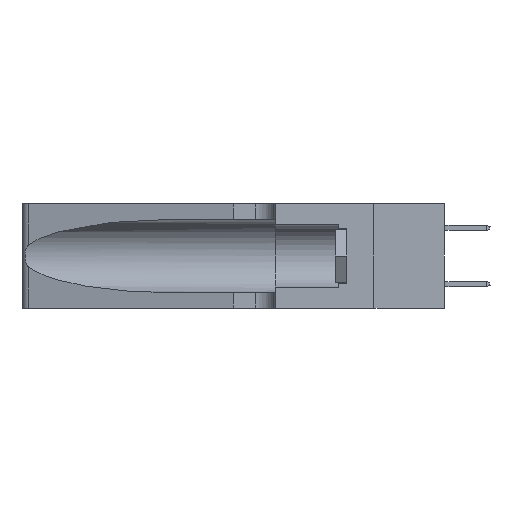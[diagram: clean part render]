
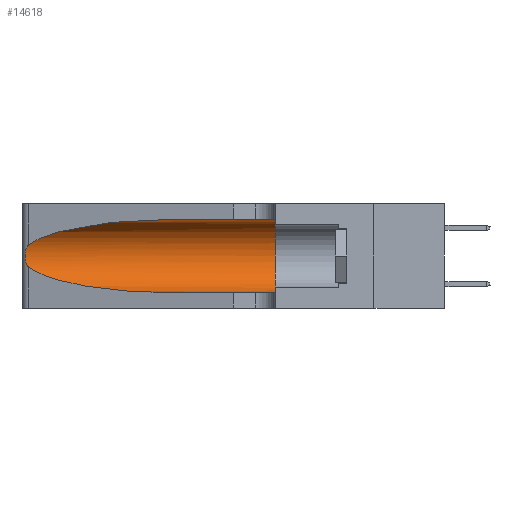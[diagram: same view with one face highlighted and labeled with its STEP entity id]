
A CAD part, left-side view. The second image highlights one B-rep face of the part: STEP entity #14618.
In plain terms, the highlighted cylindrical face has radius 3.308 mm (diameter 6.617 mm), a partial arc.
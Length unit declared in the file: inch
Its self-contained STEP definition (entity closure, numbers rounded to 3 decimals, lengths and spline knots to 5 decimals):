
#672 = CYLINDRICAL_SURFACE ( 'NONE', #8063, 0.13025 ) ;
#732 = CARTESIAN_POINT ( 'NONE',  ( 0.25789, 1.23486, 0.15765 ) ) ;
#1473 = VERTEX_POINT ( 'NONE', #19473 ) ;
#2436 = CARTESIAN_POINT ( 'NONE',  ( 0.25487, 1.22718, 0.22369 ) ) ;
#3015 = ORIENTED_EDGE ( 'NONE', *, *, #11778, .T. ) ;
#3495 = CARTESIAN_POINT ( 'NONE',  ( 0.25555, 1.22993, 0.14849 ) ) ;
#3875 = LINE ( 'NONE', #29066, #17285 ) ;
#5190 = ORIENTED_EDGE ( 'NONE', *, *, #21490, .F. ) ;
#5998 = ORIENTED_EDGE ( 'NONE', *, *, #27264, .F. ) ;
#6663 = VERTEX_POINT ( 'NONE', #19026 ) ;
#7786 = CARTESIAN_POINT ( 'NONE',  ( 0.1305, 0.72297, 0.05475 ) ) ;
#7862 = EDGE_CURVE ( 'NONE', #17977, #1473, #10092, .T. ) ;
#8063 = AXIS2_PLACEMENT_3D ( 'NONE', #27535, #8978, #30194 ) ;
#8717 = CIRCLE ( 'NONE', #23995, 0.13025 ) ;
#8726 = CARTESIAN_POINT ( 'NONE',  ( 0.25555, 1.22994, 0.2215 ) ) ;
#8837 = CARTESIAN_POINT ( 'NONE',  ( 0.25787, 1.23484, 0.2124 ) ) ;
#8978 = DIRECTION ( 'NONE',  ( 0., -1., 0. ) ) ;
#10092 =( BOUNDED_CURVE ( )  B_SPLINE_CURVE ( 3, ( #31660, #34314, #18511, #2436 ),
 .UNSPECIFIED., .F., .T. ) 
 B_SPLINE_CURVE_WITH_KNOTS ( ( 4, 4 ),
 ( 1.5708, 2.84003 ),
 .UNSPECIFIED. ) 
 CURVE ( )  GEOMETRIC_REPRESENTATION_ITEM ( )  RATIONAL_B_SPLINE_CURVE ( ( 1., 0.87, 0.87, 1. ) ) 
 REPRESENTATION_ITEM ( '' )  );
#10365 = ORIENTED_EDGE ( 'NONE', *, *, #31930, .T. ) ;
#10540 = DIRECTION ( 'NONE',  ( 0., -1., 0. ) ) ;
#11531 = CARTESIAN_POINT ( 'NONE',  ( 0.26018, 1.23835, 0.19895 ) ) ;
#11778 = EDGE_CURVE ( 'NONE', #1473, #6663, #19892, .T. ) ;
#11958 = CARTESIAN_POINT ( 'NONE',  ( 0.1305, 0.35, 0.185 ) ) ;
#14196 = CARTESIAN_POINT ( 'NONE',  ( 0.26075, 1.23896, 0.178 ) ) ;
#14613 = DIRECTION ( 'NONE',  ( 0., 0., 1. ) ) ;
#14618 = ADVANCED_FACE ( 'NONE', ( #22096 ), #672, .F. ) ;
#15187 = CARTESIAN_POINT ( 'NONE',  ( 0.1305, 1.61858, 0.31525 ) ) ;
#16752 = CARTESIAN_POINT ( 'NONE',  ( 0.25487, 1.22718, 0.22369 ) ) ;
#16816 = LINE ( 'NONE', #15187, #30063 ) ;
#16869 = CARTESIAN_POINT ( 'NONE',  ( 0.25856, 1.23593, 0.16098 ) ) ;
#16900 = CARTESIAN_POINT ( 'NONE',  ( 0.1305, 0.72297, 0.31525 ) ) ;
#17285 = VECTOR ( 'NONE', #10540, 39.37008 ) ;
#17691 = EDGE_CURVE ( 'NONE', #20836, #21508, #3875, .T. ) ;
#17977 = VERTEX_POINT ( 'NONE', #16900 ) ;
#18511 = CARTESIAN_POINT ( 'NONE',  ( 0.2373, 1.15595, 0.28018 ) ) ;
#19026 = CARTESIAN_POINT ( 'NONE',  ( 0.25487, 1.22718, 0.14631 ) ) ;
#19473 = CARTESIAN_POINT ( 'NONE',  ( 0.25487, 1.22718, 0.22369 ) ) ;
#19544 = CARTESIAN_POINT ( 'NONE',  ( 0.25639, 1.23186, 0.15144 ) ) ;
#19892 = B_SPLINE_CURVE_WITH_KNOTS ( 'NONE', 3,
 ( #16752, #8726, #24770, #8837, #27398, #11531, #30056, #14196, #32678, #16869, #732, #19544, #3495, #22223 ),
 .UNSPECIFIED., .F., .F.,
 ( 4, 2, 2, 2, 2, 2, 4 ),
 ( 0., 0.00027, 0.00053, 0.00107, 0.0016, 0.00187, 0.00214 ),
 .UNSPECIFIED. ) ;
#19973 = CARTESIAN_POINT ( 'NONE',  ( 0.1305, 0.35, 0.05475 ) ) ;
#20836 = VERTEX_POINT ( 'NONE', #25857 ) ;
#21490 = EDGE_CURVE ( 'NONE', #33647, #21508, #8717, .T. ) ;
#21508 = VERTEX_POINT ( 'NONE', #19973 ) ;
#22096 = FACE_OUTER_BOUND ( 'NONE', #29801, .T. ) ;
#22223 = CARTESIAN_POINT ( 'NONE',  ( 0.25487, 1.22718, 0.14631 ) ) ;
#23511 =( BOUNDED_CURVE ( )  B_SPLINE_CURVE ( 3, ( #31550, #34200, #23721, #7786 ),
 .UNSPECIFIED., .F., .T. ) 
 B_SPLINE_CURVE_WITH_KNOTS ( ( 4, 4 ),
 ( 3.44316, 4.71239 ),
 .UNSPECIFIED. ) 
 CURVE ( )  GEOMETRIC_REPRESENTATION_ITEM ( )  RATIONAL_B_SPLINE_CURVE ( ( 1., 0.87, 0.87, 1. ) ) 
 REPRESENTATION_ITEM ( '' )  );
#23721 = CARTESIAN_POINT ( 'NONE',  ( 0.18966, 0.96281, 0.05475 ) ) ;
#23995 = AXIS2_PLACEMENT_3D ( 'NONE', #11958, #30481, #14613 ) ;
#24034 = ORIENTED_EDGE ( 'NONE', *, *, #7862, .T. ) ;
#24770 = CARTESIAN_POINT ( 'NONE',  ( 0.25639, 1.23184, 0.21858 ) ) ;
#25688 = ORIENTED_EDGE ( 'NONE', *, *, #17691, .T. ) ;
#25857 = CARTESIAN_POINT ( 'NONE',  ( 0.1305, 0.72297, 0.05475 ) ) ;
#27264 = EDGE_CURVE ( 'NONE', #17977, #33647, #16816, .T. ) ;
#27398 = CARTESIAN_POINT ( 'NONE',  ( 0.25854, 1.2359, 0.20912 ) ) ;
#27535 = CARTESIAN_POINT ( 'NONE',  ( 0.1305, 1.61858, 0.185 ) ) ;
#29066 = CARTESIAN_POINT ( 'NONE',  ( 0.1305, 1.61858, 0.05475 ) ) ;
#29801 = EDGE_LOOP ( 'NONE', ( #24034, #3015, #10365, #25688, #5190, #5998 ) ) ;
#30056 = CARTESIAN_POINT ( 'NONE',  ( 0.26075, 1.23896, 0.19203 ) ) ;
#30059 = CARTESIAN_POINT ( 'NONE',  ( 0.1305, 0.35, 0.31525 ) ) ;
#30063 = VECTOR ( 'NONE', #33668, 39.37008 ) ;
#30194 = DIRECTION ( 'NONE',  ( 0., 0., -1. ) ) ;
#30481 = DIRECTION ( 'NONE',  ( 0., 1., 0. ) ) ;
#31550 = CARTESIAN_POINT ( 'NONE',  ( 0.25487, 1.22718, 0.14631 ) ) ;
#31660 = CARTESIAN_POINT ( 'NONE',  ( 0.1305, 0.72297, 0.31525 ) ) ;
#31930 = EDGE_CURVE ( 'NONE', #6663, #20836, #23511, .T. ) ;
#32678 = CARTESIAN_POINT ( 'NONE',  ( 0.26017, 1.23833, 0.17102 ) ) ;
#33647 = VERTEX_POINT ( 'NONE', #30059 ) ;
#33668 = DIRECTION ( 'NONE',  ( 0., -1., 0. ) ) ;
#34200 = CARTESIAN_POINT ( 'NONE',  ( 0.2373, 1.15595, 0.08982 ) ) ;
#34314 = CARTESIAN_POINT ( 'NONE',  ( 0.18966, 0.96281, 0.31525 ) ) ;
